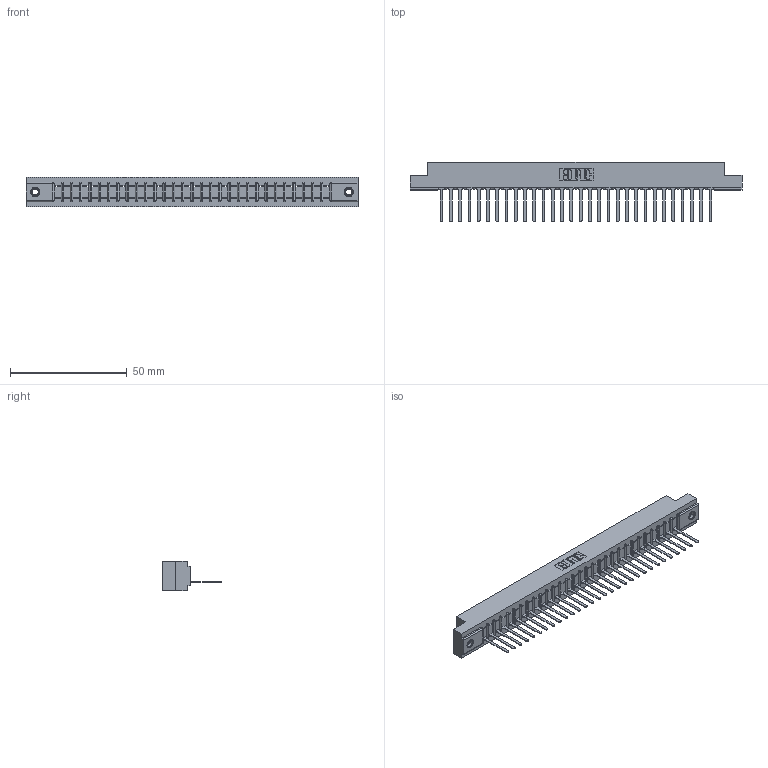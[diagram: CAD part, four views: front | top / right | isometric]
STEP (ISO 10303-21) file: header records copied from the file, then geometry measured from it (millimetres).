
FILE_DESCRIPTION (( 'STEP AP203' ), '1' );
FILE_NAME ('357-030-547-107.STEP', '2019-09-14T04:18:59', ( '' ), ( '' ), 'SwSTEP 2.0', 'SolidWorks 2016', '' );
FILE_SCHEMA (( 'CONFIG_CONTROL_DESIGN' ));
Length unit declared in the file: inch
Products named in the file (4): 307-290-001_547; 357-030-547-107; 345-250-001_345-250-005-103; 307 Part_.156 Dia Mounting Holes
Assembly tree (33 placements, depth 2):
  357-030-547-107
    307 Part_.156 Dia Mounting Holes
    307-290-001_547  x30
    345-250-001_345-250-005-103  x2
Bounding box: 141.88 x 25.43 x 12.7 mm (x, y, z)
Volume: 14716.7 mm3; surface area: 15911.1 mm2
Topology: 33 solids, 33 shells, 1889 faces, 5319 edges, 3414 vertices
Faces by surface type: plane 1212, cylinder 599, sphere 62, cone 12, torus 4
Entity records: 28351 total; most frequent: CARTESIAN_POINT 4751, ORIENTED_EDGE 4730, DIRECTION 4637, EDGE_CURVE 2365, LINE 1809, VECTOR 1809, VERTEX_POINT 1528, AXIS2_PLACEMENT_3D 1414
